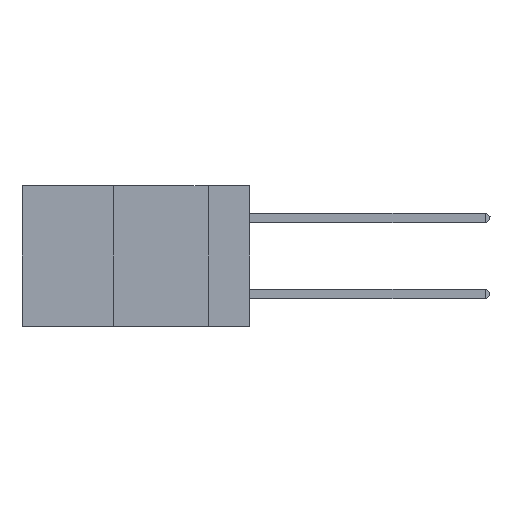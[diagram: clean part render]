
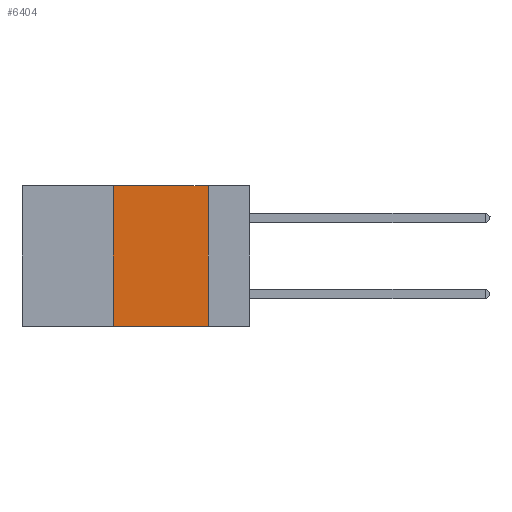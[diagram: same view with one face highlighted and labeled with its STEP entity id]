
A CAD part, left-side view. The second image highlights one B-rep face of the part: STEP entity #6404.
In plain terms, the highlighted planar face has unit normal (-1, 0, 0).
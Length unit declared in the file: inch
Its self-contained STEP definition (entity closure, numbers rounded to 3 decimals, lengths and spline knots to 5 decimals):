
#339 = EDGE_CURVE ( 'NONE', #21649, #14203, #18174, .T. ) ;
#425 = LINE ( 'NONE', #21379, #4924 ) ;
#675 = VECTOR ( 'NONE', #14414, 39.37008 ) ;
#857 = DIRECTION ( 'NONE',  ( 0., 0., -1. ) ) ;
#3377 = VECTOR ( 'NONE', #14119, 39.37008 ) ;
#4443 = VERTEX_POINT ( 'NONE', #21077 ) ;
#4924 = VECTOR ( 'NONE', #12440, 39.37008 ) ;
#5138 = VECTOR ( 'NONE', #13852, 39.37008 ) ;
#5827 = ORIENTED_EDGE ( 'NONE', *, *, #21947, .F. ) ;
#5850 = ORIENTED_EDGE ( 'NONE', *, *, #11105, .F. ) ;
#6056 = ORIENTED_EDGE ( 'NONE', *, *, #17586, .F. ) ;
#6404 = ADVANCED_FACE ( 'NONE', ( #6600 ), #21214, .F. ) ;
#6600 = FACE_OUTER_BOUND ( 'NONE', #12469, .T. ) ;
#6758 = ORIENTED_EDGE ( 'NONE', *, *, #339, .T. ) ;
#7072 = CARTESIAN_POINT ( 'NONE',  ( 0., 0.6, -0.37 ) ) ;
#8430 = VERTEX_POINT ( 'NONE', #12330 ) ;
#10162 = CARTESIAN_POINT ( 'NONE',  ( 0., 0.11, -0.37 ) ) ;
#10342 = CARTESIAN_POINT ( 'NONE',  ( 0., 0.6, 0. ) ) ;
#10766 = LINE ( 'NONE', #23344, #675 ) ;
#10938 = AXIS2_PLACEMENT_3D ( 'NONE', #10342, #12184, #857 ) ;
#11105 = EDGE_CURVE ( 'NONE', #4443, #8430, #10766, .T. ) ;
#12010 = CARTESIAN_POINT ( 'NONE',  ( 0., 0.11, 0. ) ) ;
#12184 = DIRECTION ( 'NONE',  ( 1., 0., 0. ) ) ;
#12330 = CARTESIAN_POINT ( 'NONE',  ( 0., 0.11, 0. ) ) ;
#12440 = DIRECTION ( 'NONE',  ( 0., 0., 1. ) ) ;
#12469 = EDGE_LOOP ( 'NONE', ( #5827, #5850, #6056, #6758 ) ) ;
#13852 = DIRECTION ( 'NONE',  ( 0., 0., -1. ) ) ;
#14119 = DIRECTION ( 'NONE',  ( 0., -1., 0. ) ) ;
#14203 = VERTEX_POINT ( 'NONE', #10162 ) ;
#14414 = DIRECTION ( 'NONE',  ( 0., -1., 0. ) ) ;
#17586 = EDGE_CURVE ( 'NONE', #21649, #4443, #425, .T. ) ;
#18174 = LINE ( 'NONE', #7072, #3377 ) ;
#19269 = LINE ( 'NONE', #12010, #5138 ) ;
#20211 = CARTESIAN_POINT ( 'NONE',  ( 0., 0.36, -0.37 ) ) ;
#21077 = CARTESIAN_POINT ( 'NONE',  ( 0., 0.36, 0. ) ) ;
#21214 = PLANE ( 'NONE',  #10938 ) ;
#21379 = CARTESIAN_POINT ( 'NONE',  ( 0., 0.36, 0. ) ) ;
#21649 = VERTEX_POINT ( 'NONE', #20211 ) ;
#21947 = EDGE_CURVE ( 'NONE', #8430, #14203, #19269, .T. ) ;
#23344 = CARTESIAN_POINT ( 'NONE',  ( 0., 0.6, 0. ) ) ;
